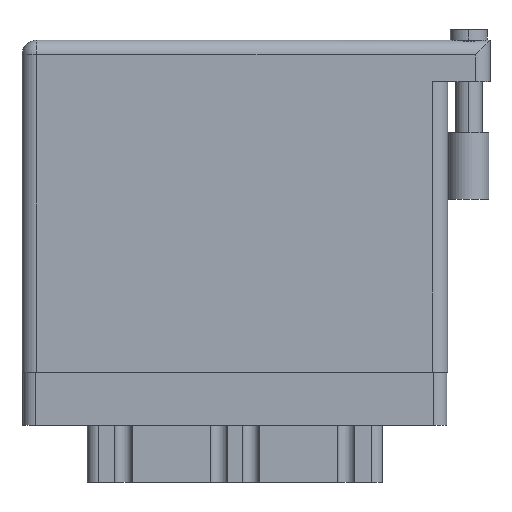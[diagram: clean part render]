
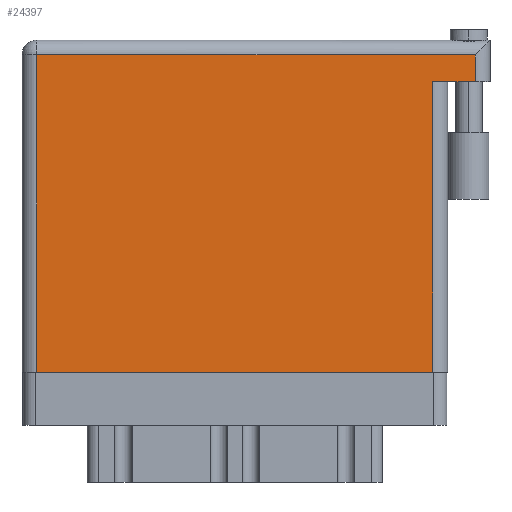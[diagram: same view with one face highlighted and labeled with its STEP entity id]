
A CAD part, front view. The second image highlights one B-rep face of the part: STEP entity #24397.
In plain terms, the highlighted face is planar.
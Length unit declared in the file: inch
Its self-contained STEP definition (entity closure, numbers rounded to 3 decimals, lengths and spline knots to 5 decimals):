
#18 = PLANE ( 'NONE',  #21478 ) ;
#3036 = DIRECTION ( 'NONE',  ( 0., 1., 0. ) ) ;
#3100 = ORIENTED_EDGE ( 'NONE', *, *, #14911, .T. ) ;
#3902 = LINE ( 'NONE', #14488, #16177 ) ;
#4064 = VECTOR ( 'NONE', #13635, 39.37008 ) ;
#4567 = EDGE_LOOP ( 'NONE', ( #11775, #3100, #13295, #21916, #11381, #15194 ) ) ;
#6070 = VERTEX_POINT ( 'NONE', #27269 ) ;
#7070 = CARTESIAN_POINT ( 'NONE',  ( 2.208, 1.369, 0. ) ) ;
#9323 = CARTESIAN_POINT ( 'NONE',  ( 1.938, 1.369, 0. ) ) ;
#9411 = CARTESIAN_POINT ( 'NONE',  ( 2.138, 1.369, 0. ) ) ;
#9849 = DIRECTION ( 'NONE',  ( -1., 0., 0. ) ) ;
#10855 = CARTESIAN_POINT ( 'NONE',  ( 2.138, 1.566, 0. ) ) ;
#11264 = VECTOR ( 'NONE', #22551, 39.37008 ) ;
#11381 = ORIENTED_EDGE ( 'NONE', *, *, #18690, .T. ) ;
#11775 = ORIENTED_EDGE ( 'NONE', *, *, #12178, .T. ) ;
#12178 = EDGE_CURVE ( 'NONE', #30677, #33286, #13972, .T. ) ;
#13295 = ORIENTED_EDGE ( 'NONE', *, *, #23185, .F. ) ;
#13635 = DIRECTION ( 'NONE',  ( 1., 0., 0. ) ) ;
#13972 = LINE ( 'NONE', #24768, #4064 ) ;
#14488 = CARTESIAN_POINT ( 'NONE',  ( 0., 1.496, 0. ) ) ;
#14911 = EDGE_CURVE ( 'NONE', #33286, #6070, #17656, .T. ) ;
#15105 = CARTESIAN_POINT ( 'NONE',  ( 0.07, 0., 0. ) ) ;
#15194 = ORIENTED_EDGE ( 'NONE', *, *, #24663, .T. ) ;
#16177 = VECTOR ( 'NONE', #20214, 39.37008 ) ;
#17054 = CARTESIAN_POINT ( 'NONE',  ( 1.938, 0., 0. ) ) ;
#17417 = VECTOR ( 'NONE', #9849, 39.37008 ) ;
#17656 = LINE ( 'NONE', #9323, #11264 ) ;
#17665 = CARTESIAN_POINT ( 'NONE',  ( 2.138, 1.496, 0. ) ) ;
#17836 = LINE ( 'NONE', #7070, #17417 ) ;
#17881 = DIRECTION ( 'NONE',  ( 0., -1., 0. ) ) ;
#18690 = EDGE_CURVE ( 'NONE', #22011, #23263, #3902, .T. ) ;
#19471 = DIRECTION ( 'NONE',  ( 0., 0., -1. ) ) ;
#20214 = DIRECTION ( 'NONE',  ( -1., 0., 0. ) ) ;
#20366 = VERTEX_POINT ( 'NONE', #9411 ) ;
#21478 = AXIS2_PLACEMENT_3D ( 'NONE', #25378, #19471, #27801 ) ;
#21805 = LINE ( 'NONE', #10855, #26499 ) ;
#21916 = ORIENTED_EDGE ( 'NONE', *, *, #32752, .T. ) ;
#22011 = VERTEX_POINT ( 'NONE', #17665 ) ;
#22551 = DIRECTION ( 'NONE',  ( 0., 1., 0. ) ) ;
#23185 = EDGE_CURVE ( 'NONE', #20366, #6070, #17836, .T. ) ;
#23263 = VERTEX_POINT ( 'NONE', #25848 ) ;
#23462 = LINE ( 'NONE', #15105, #29249 ) ;
#23844 = FACE_OUTER_BOUND ( 'NONE', #4567, .T. ) ;
#24326 = CARTESIAN_POINT ( 'NONE',  ( 0.07, 0., 0. ) ) ;
#24397 = ADVANCED_FACE ( 'NONE', ( #23844 ), #18, .F. ) ;
#24663 = EDGE_CURVE ( 'NONE', #23263, #30677, #23462, .T. ) ;
#24768 = CARTESIAN_POINT ( 'NONE',  ( 0., 0., 0. ) ) ;
#25378 = CARTESIAN_POINT ( 'NONE',  ( 0., 1.566, 0. ) ) ;
#25848 = CARTESIAN_POINT ( 'NONE',  ( 0.07, 1.496, 0. ) ) ;
#26499 = VECTOR ( 'NONE', #3036, 39.37008 ) ;
#27269 = CARTESIAN_POINT ( 'NONE',  ( 1.938, 1.369, 0. ) ) ;
#27801 = DIRECTION ( 'NONE',  ( -1., 0., 0. ) ) ;
#29249 = VECTOR ( 'NONE', #17881, 39.37008 ) ;
#30677 = VERTEX_POINT ( 'NONE', #24326 ) ;
#32752 = EDGE_CURVE ( 'NONE', #20366, #22011, #21805, .T. ) ;
#33286 = VERTEX_POINT ( 'NONE', #17054 ) ;
